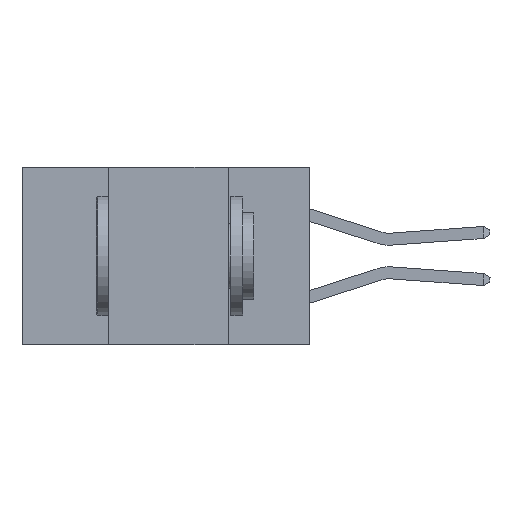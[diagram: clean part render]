
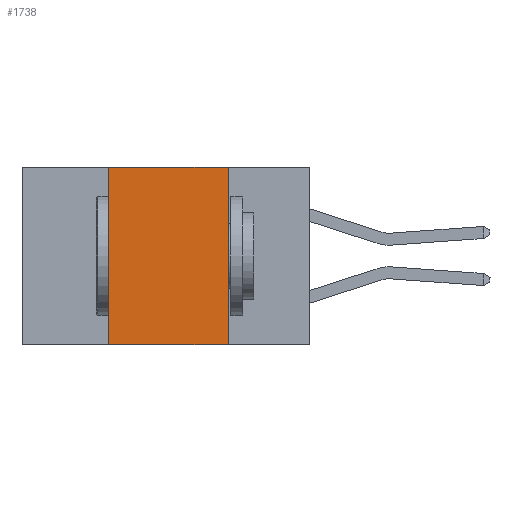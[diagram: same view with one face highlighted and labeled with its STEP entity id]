
A CAD part, left-side view. The second image highlights one B-rep face of the part: STEP entity #1738.
In plain terms, the highlighted planar face has unit normal (-1, 0, 0).
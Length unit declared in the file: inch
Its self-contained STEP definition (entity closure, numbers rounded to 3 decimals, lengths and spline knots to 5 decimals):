
#24 = LINE ( 'NONE', #5842, #1381 ) ;
#728 = DIRECTION ( 'NONE',  ( 1., 0., 0. ) ) ;
#1265 = CARTESIAN_POINT ( 'NONE',  ( 0., 0.42, 0. ) ) ;
#1381 = VECTOR ( 'NONE', #21505, 39.37008 ) ;
#1738 = ADVANCED_FACE ( 'NONE', ( #27638 ), #9388, .F. ) ;
#1902 = VECTOR ( 'NONE', #20307, 39.37008 ) ;
#2326 = EDGE_CURVE ( 'NONE', #5851, #18903, #5239, .T. ) ;
#3119 = VECTOR ( 'NONE', #28219, 39.37008 ) ;
#3349 = CARTESIAN_POINT ( 'NONE',  ( 0., 0.6, -0.37 ) ) ;
#3760 = VERTEX_POINT ( 'NONE', #28371 ) ;
#4457 = EDGE_CURVE ( 'NONE', #7974, #5851, #10695, .T. ) ;
#5043 = DIRECTION ( 'NONE',  ( 0., 0., -1. ) ) ;
#5136 = CARTESIAN_POINT ( 'NONE',  ( 0., 0.6, 0. ) ) ;
#5161 = LINE ( 'NONE', #3349, #18130 ) ;
#5239 = LINE ( 'NONE', #8201, #3119 ) ;
#5842 = CARTESIAN_POINT ( 'NONE',  ( 0., 0.42, 0. ) ) ;
#5851 = VERTEX_POINT ( 'NONE', #27774 ) ;
#7974 = VERTEX_POINT ( 'NONE', #1265 ) ;
#8201 = CARTESIAN_POINT ( 'NONE',  ( 0., 0.17, 0. ) ) ;
#9388 = PLANE ( 'NONE',  #13317 ) ;
#10695 = LINE ( 'NONE', #24801, #1902 ) ;
#12505 = ORIENTED_EDGE ( 'NONE', *, *, #20947, .T. ) ;
#13317 = AXIS2_PLACEMENT_3D ( 'NONE', #5136, #728, #5043 ) ;
#14405 = CARTESIAN_POINT ( 'NONE',  ( 0., 0.17, -0.37 ) ) ;
#14696 = DIRECTION ( 'NONE',  ( 0., -1., 0. ) ) ;
#18130 = VECTOR ( 'NONE', #14696, 39.37008 ) ;
#18750 = ORIENTED_EDGE ( 'NONE', *, *, #26638, .F. ) ;
#18861 = EDGE_LOOP ( 'NONE', ( #19711, #23424, #18750, #12505 ) ) ;
#18903 = VERTEX_POINT ( 'NONE', #14405 ) ;
#19711 = ORIENTED_EDGE ( 'NONE', *, *, #2326, .F. ) ;
#20307 = DIRECTION ( 'NONE',  ( 0., -1., 0. ) ) ;
#20947 = EDGE_CURVE ( 'NONE', #3760, #18903, #5161, .T. ) ;
#21505 = DIRECTION ( 'NONE',  ( 0., 0., 1. ) ) ;
#23424 = ORIENTED_EDGE ( 'NONE', *, *, #4457, .F. ) ;
#24801 = CARTESIAN_POINT ( 'NONE',  ( 0., 0.6, 0. ) ) ;
#26638 = EDGE_CURVE ( 'NONE', #3760, #7974, #24, .T. ) ;
#27638 = FACE_OUTER_BOUND ( 'NONE', #18861, .T. ) ;
#27774 = CARTESIAN_POINT ( 'NONE',  ( 0., 0.17, 0. ) ) ;
#28219 = DIRECTION ( 'NONE',  ( 0., 0., -1. ) ) ;
#28371 = CARTESIAN_POINT ( 'NONE',  ( 0., 0.42, -0.37 ) ) ;
